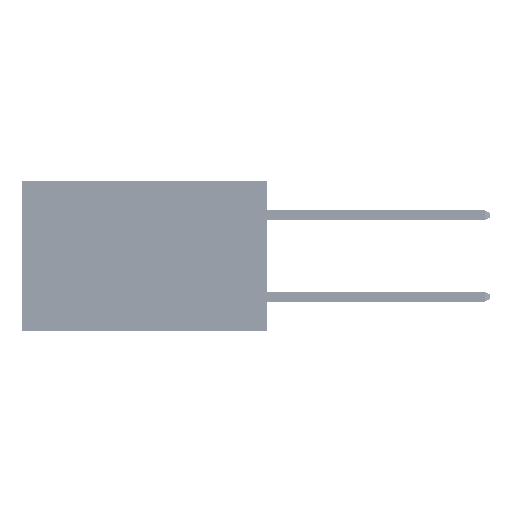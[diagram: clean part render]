
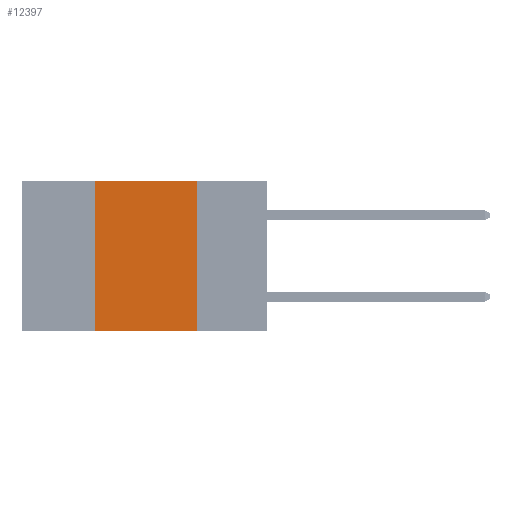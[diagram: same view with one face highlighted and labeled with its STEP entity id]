
A CAD part, left-side view. The second image highlights one B-rep face of the part: STEP entity #12397.
In plain terms, the highlighted planar face has unit normal (-1, 0, 0).
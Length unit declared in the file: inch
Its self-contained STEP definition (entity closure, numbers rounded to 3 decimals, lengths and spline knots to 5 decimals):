
#1962 = ORIENTED_EDGE ( 'NONE', *, *, #34310, .F. ) ;
#5475 = CARTESIAN_POINT ( 'NONE',  ( 0., 0.17, 0. ) ) ;
#5541 = CARTESIAN_POINT ( 'NONE',  ( 0., 0.6, -0.37 ) ) ;
#5778 = CARTESIAN_POINT ( 'NONE',  ( 0., 0.42, -0.37 ) ) ;
#5921 = LINE ( 'NONE', #47181, #31803 ) ;
#5992 = VECTOR ( 'NONE', #31580, 39.37008 ) ;
#6718 = DIRECTION ( 'NONE',  ( 0., -1., 0. ) ) ;
#7639 = DIRECTION ( 'NONE',  ( 1., 0., 0. ) ) ;
#8302 = CARTESIAN_POINT ( 'NONE',  ( 0., 0.42, 0. ) ) ;
#8740 = LINE ( 'NONE', #5541, #5992 ) ;
#12397 = ADVANCED_FACE ( 'NONE', ( #25789 ), #40301, .F. ) ;
#13181 = VECTOR ( 'NONE', #6718, 39.37008 ) ;
#14975 = EDGE_CURVE ( 'NONE', #15012, #20158, #8740, .T. ) ;
#15012 = VERTEX_POINT ( 'NONE', #5778 ) ;
#16945 = VERTEX_POINT ( 'NONE', #8302 ) ;
#18194 = CARTESIAN_POINT ( 'NONE',  ( 0., 0.42, 0. ) ) ;
#20158 = VERTEX_POINT ( 'NONE', #48363 ) ;
#20644 = DIRECTION ( 'NONE',  ( 0., 0., -1. ) ) ;
#22105 = DIRECTION ( 'NONE',  ( 0., 0., -1. ) ) ;
#25789 = FACE_OUTER_BOUND ( 'NONE', #43053, .T. ) ;
#28738 = ORIENTED_EDGE ( 'NONE', *, *, #31874, .F. ) ;
#30101 = VECTOR ( 'NONE', #33194, 39.37008 ) ;
#31442 = VERTEX_POINT ( 'NONE', #5475 ) ;
#31580 = DIRECTION ( 'NONE',  ( 0., -1., 0. ) ) ;
#31803 = VECTOR ( 'NONE', #20644, 39.37008 ) ;
#31874 = EDGE_CURVE ( 'NONE', #15012, #16945, #36866, .T. ) ;
#32945 = CARTESIAN_POINT ( 'NONE',  ( 0., 0.6, 0. ) ) ;
#33194 = DIRECTION ( 'NONE',  ( 0., 0., 1. ) ) ;
#33479 = LINE ( 'NONE', #40354, #13181 ) ;
#34310 = EDGE_CURVE ( 'NONE', #31442, #20158, #5921, .T. ) ;
#35304 = ORIENTED_EDGE ( 'NONE', *, *, #14975, .T. ) ;
#36866 = LINE ( 'NONE', #18194, #30101 ) ;
#40301 = PLANE ( 'NONE',  #43529 ) ;
#40354 = CARTESIAN_POINT ( 'NONE',  ( 0., 0.6, 0. ) ) ;
#42521 = ORIENTED_EDGE ( 'NONE', *, *, #45417, .F. ) ;
#43053 = EDGE_LOOP ( 'NONE', ( #1962, #42521, #28738, #35304 ) ) ;
#43529 = AXIS2_PLACEMENT_3D ( 'NONE', #32945, #7639, #22105 ) ;
#45417 = EDGE_CURVE ( 'NONE', #16945, #31442, #33479, .T. ) ;
#47181 = CARTESIAN_POINT ( 'NONE',  ( 0., 0.17, 0. ) ) ;
#48363 = CARTESIAN_POINT ( 'NONE',  ( 0., 0.17, -0.37 ) ) ;
